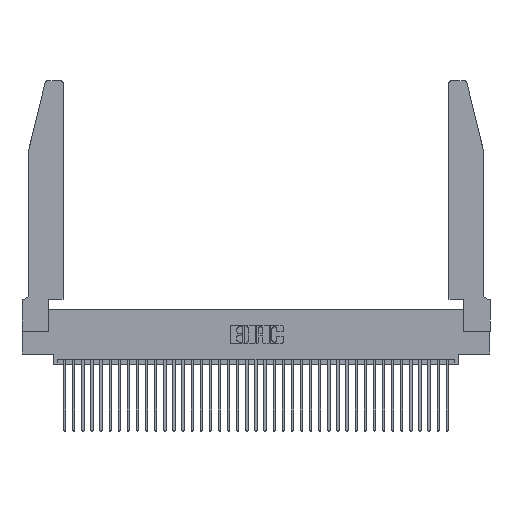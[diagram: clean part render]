
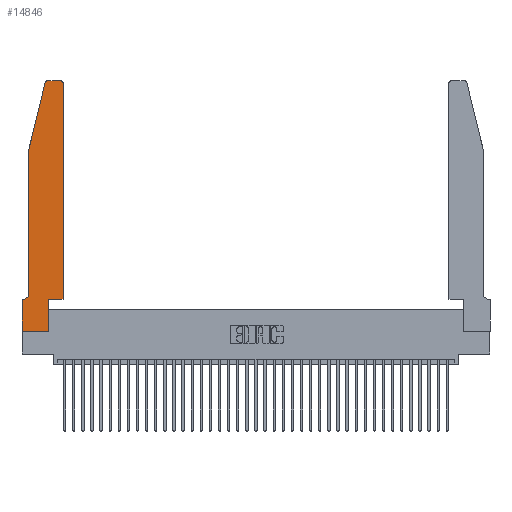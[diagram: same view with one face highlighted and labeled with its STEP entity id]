
A CAD part, top view. The second image highlights one B-rep face of the part: STEP entity #14846.
In plain terms, the highlighted planar face has unit normal (0, 0, 1).
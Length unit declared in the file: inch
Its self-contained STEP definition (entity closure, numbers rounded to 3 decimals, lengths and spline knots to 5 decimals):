
#30 = CARTESIAN_POINT ( 'NONE',  ( 0.2605, 2.75, 0.37 ) ) ;
#733 = LINE ( 'NONE', #9678, #7781 ) ;
#998 = LINE ( 'NONE', #35122, #24825 ) ;
#1460 = EDGE_CURVE ( 'NONE', #38135, #20576, #1825, .T. ) ;
#1516 = EDGE_CURVE ( 'NONE', #36676, #36232, #21914, .T. ) ;
#1688 = CARTESIAN_POINT ( 'NONE',  ( 0., 0., 0.37 ) ) ;
#1825 = CIRCLE ( 'NONE', #13023, 0.07 ) ;
#2042 = ORIENTED_EDGE ( 'NONE', *, *, #23523, .T. ) ;
#2259 = CARTESIAN_POINT ( 'NONE',  ( 0., 0.35, 0.37 ) ) ;
#2963 = DIRECTION ( 'NONE',  ( 0., 0., 1. ) ) ;
#4575 = DIRECTION ( 'NONE',  ( 0., -1., 0. ) ) ;
#5368 = EDGE_CURVE ( 'NONE', #30090, #38135, #18792, .T. ) ;
#6060 = ORIENTED_EDGE ( 'NONE', *, *, #12431, .T. ) ;
#6693 = CARTESIAN_POINT ( 'NONE',  ( 0.25487, 2.72718, 0.37 ) ) ;
#7389 = CARTESIAN_POINT ( 'NONE',  ( 0., 0., 0.37 ) ) ;
#7599 = CARTESIAN_POINT ( 'NONE',  ( 0.0755, 2., 0.37 ) ) ;
#7781 = VECTOR ( 'NONE', #12666, 39.37008 ) ;
#8194 = EDGE_CURVE ( 'NONE', #19065, #13219, #11189, .T. ) ;
#8343 = ORIENTED_EDGE ( 'NONE', *, *, #34782, .T. ) ;
#9678 = CARTESIAN_POINT ( 'NONE',  ( 0.4505, 0.35, 0.37 ) ) ;
#9812 = AXIS2_PLACEMENT_3D ( 'NONE', #12391, #33218, #15354 ) ;
#9878 = EDGE_CURVE ( 'NONE', #37841, #36676, #733, .T. ) ;
#11181 = LINE ( 'NONE', #13780, #26075 ) ;
#11189 = LINE ( 'NONE', #37788, #12140 ) ;
#11530 = CARTESIAN_POINT ( 'NONE',  ( 0.0755, 2., 0.37 ) ) ;
#11811 = VERTEX_POINT ( 'NONE', #6693 ) ;
#12127 = CIRCLE ( 'NONE', #9812, 0.03 ) ;
#12140 = VECTOR ( 'NONE', #17032, 39.37008 ) ;
#12348 = CARTESIAN_POINT ( 'NONE',  ( 0.0755, 0.42, 0.37 ) ) ;
#12391 = CARTESIAN_POINT ( 'NONE',  ( 0.284, 2.72, 0.37 ) ) ;
#12431 = EDGE_CURVE ( 'NONE', #13609, #11811, #12127, .T. ) ;
#12666 = DIRECTION ( 'NONE',  ( 0., 1., 0. ) ) ;
#13023 = AXIS2_PLACEMENT_3D ( 'NONE', #32441, #14559, #35375 ) ;
#13096 = CARTESIAN_POINT ( 'NONE',  ( 0.4205, 2.75, 0.37 ) ) ;
#13219 = VERTEX_POINT ( 'NONE', #24551 ) ;
#13420 = EDGE_LOOP ( 'NONE', ( #2042, #6060, #8343, #15946, #29319, #36127, #32545, #29576, #15046, #16893, #29744, #23752 ) ) ;
#13609 = VERTEX_POINT ( 'NONE', #23912 ) ;
#13780 = CARTESIAN_POINT ( 'NONE',  ( 0., 0., 0.37 ) ) ;
#14305 = DIRECTION ( 'NONE',  ( 1., 0., 0. ) ) ;
#14559 = DIRECTION ( 'NONE',  ( 0., 0., -1. ) ) ;
#14846 = ADVANCED_FACE ( 'NONE', ( #38427 ), #32129, .T. ) ;
#15046 = ORIENTED_EDGE ( 'NONE', *, *, #8194, .T. ) ;
#15354 = DIRECTION ( 'NONE',  ( 1., 0., 0. ) ) ;
#15946 = ORIENTED_EDGE ( 'NONE', *, *, #5368, .T. ) ;
#16768 = DIRECTION ( 'NONE',  ( 1., 0., 0. ) ) ;
#16893 = ORIENTED_EDGE ( 'NONE', *, *, #20001, .T. ) ;
#17032 = DIRECTION ( 'NONE',  ( 0., 1., 0. ) ) ;
#17149 = VECTOR ( 'NONE', #33724, 39.37008 ) ;
#17250 = DIRECTION ( 'NONE',  ( 1., 0., 0. ) ) ;
#17353 = EDGE_CURVE ( 'NONE', #26401, #27590, #27778, .T. ) ;
#18792 = LINE ( 'NONE', #7599, #25767 ) ;
#19065 = VERTEX_POINT ( 'NONE', #19348 ) ;
#19348 = CARTESIAN_POINT ( 'NONE',  ( 0.2865, 0., 0.37 ) ) ;
#20001 = EDGE_CURVE ( 'NONE', #13219, #37841, #998, .T. ) ;
#20576 = VERTEX_POINT ( 'NONE', #32282 ) ;
#20782 = LINE ( 'NONE', #11530, #28688 ) ;
#20850 = CARTESIAN_POINT ( 'NONE',  ( 0.4205, 2.72, 0.37 ) ) ;
#21768 = CARTESIAN_POINT ( 'NONE',  ( 0.0755, 0.35, 0.37 ) ) ;
#21914 = CIRCLE ( 'NONE', #23040, 0.03 ) ;
#23040 = AXIS2_PLACEMENT_3D ( 'NONE', #20850, #2963, #23859 ) ;
#23523 = EDGE_CURVE ( 'NONE', #36232, #13609, #35713, .T. ) ;
#23752 = ORIENTED_EDGE ( 'NONE', *, *, #1516, .T. ) ;
#23859 = DIRECTION ( 'NONE',  ( 1., 0., 0. ) ) ;
#23912 = CARTESIAN_POINT ( 'NONE',  ( 0.284, 2.75, 0.37 ) ) ;
#23960 = DIRECTION ( 'NONE',  ( -1., 0., 0. ) ) ;
#24551 = CARTESIAN_POINT ( 'NONE',  ( 0.2865, 0.35, 0.37 ) ) ;
#24825 = VECTOR ( 'NONE', #14305, 39.37008 ) ;
#25100 = LINE ( 'NONE', #21768, #17149 ) ;
#25223 = DIRECTION ( 'NONE',  ( 0., -1., 0. ) ) ;
#25767 = VECTOR ( 'NONE', #4575, 39.37008 ) ;
#26075 = VECTOR ( 'NONE', #16768, 39.37008 ) ;
#26228 = CARTESIAN_POINT ( 'NONE',  ( 0.4505, 2.72, 0.37 ) ) ;
#26401 = VERTEX_POINT ( 'NONE', #30895 ) ;
#26589 = AXIS2_PLACEMENT_3D ( 'NONE', #2259, #35069, #17250 ) ;
#27590 = VERTEX_POINT ( 'NONE', #1688 ) ;
#27778 = LINE ( 'NONE', #7389, #34721 ) ;
#28688 = VECTOR ( 'NONE', #32357, 39.37008 ) ;
#29319 = ORIENTED_EDGE ( 'NONE', *, *, #1460, .T. ) ;
#29576 = ORIENTED_EDGE ( 'NONE', *, *, #33468, .T. ) ;
#29744 = ORIENTED_EDGE ( 'NONE', *, *, #9878, .T. ) ;
#30090 = VERTEX_POINT ( 'NONE', #38204 ) ;
#30895 = CARTESIAN_POINT ( 'NONE',  ( 0., 0.35, 0.37 ) ) ;
#32129 = PLANE ( 'NONE',  #26589 ) ;
#32282 = CARTESIAN_POINT ( 'NONE',  ( 0.0055, 0.35, 0.37 ) ) ;
#32357 = DIRECTION ( 'NONE',  ( -0.239, -0.971, 0. ) ) ;
#32441 = CARTESIAN_POINT ( 'NONE',  ( 0.0055, 0.42, 0.37 ) ) ;
#32545 = ORIENTED_EDGE ( 'NONE', *, *, #17353, .T. ) ;
#33218 = DIRECTION ( 'NONE',  ( 0., 0., 1. ) ) ;
#33268 = EDGE_CURVE ( 'NONE', #20576, #26401, #25100, .T. ) ;
#33468 = EDGE_CURVE ( 'NONE', #27590, #19065, #11181, .T. ) ;
#33724 = DIRECTION ( 'NONE',  ( -1., 0., 0. ) ) ;
#34721 = VECTOR ( 'NONE', #25223, 39.37008 ) ;
#34782 = EDGE_CURVE ( 'NONE', #11811, #30090, #20782, .T. ) ;
#34825 = CARTESIAN_POINT ( 'NONE',  ( 0.4505, 0.35, 0.37 ) ) ;
#35069 = DIRECTION ( 'NONE',  ( 0., 0., 1. ) ) ;
#35122 = CARTESIAN_POINT ( 'NONE',  ( 0.4505, 0.35, 0.37 ) ) ;
#35375 = DIRECTION ( 'NONE',  ( -1., 0., 0. ) ) ;
#35713 = LINE ( 'NONE', #30, #36619 ) ;
#36127 = ORIENTED_EDGE ( 'NONE', *, *, #33268, .T. ) ;
#36232 = VERTEX_POINT ( 'NONE', #13096 ) ;
#36619 = VECTOR ( 'NONE', #23960, 39.37008 ) ;
#36676 = VERTEX_POINT ( 'NONE', #26228 ) ;
#37788 = CARTESIAN_POINT ( 'NONE',  ( 0.2865, 0.35, 0.37 ) ) ;
#37841 = VERTEX_POINT ( 'NONE', #34825 ) ;
#38135 = VERTEX_POINT ( 'NONE', #12348 ) ;
#38204 = CARTESIAN_POINT ( 'NONE',  ( 0.0755, 2., 0.37 ) ) ;
#38427 = FACE_OUTER_BOUND ( 'NONE', #13420, .T. ) ;
